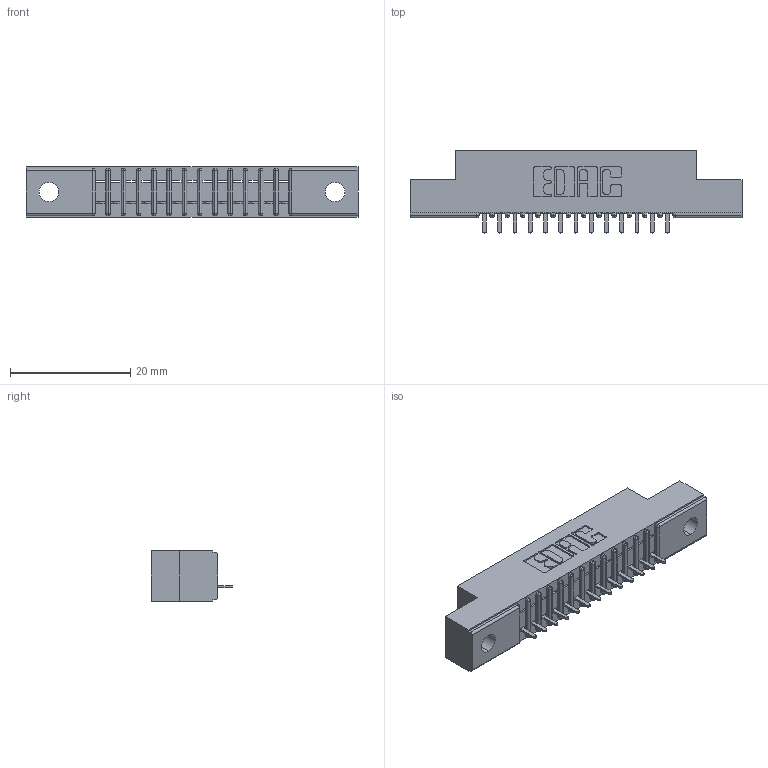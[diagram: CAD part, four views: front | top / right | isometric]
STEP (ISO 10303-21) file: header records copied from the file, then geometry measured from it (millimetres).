
FILE_DESCRIPTION (( 'STEP AP203' ), '1' );
FILE_NAME ('391-013-524-102.STEP', '2018-08-08T16:52:36', ( '' ), ( '' ), 'SwSTEP 2.0', 'SolidWorks 2016', '' );
FILE_SCHEMA (( 'CONFIG_CONTROL_DESIGN' ));
Length unit declared in the file: inch
Products named in the file (3): 391-013-524-102; 341 Part_.128 (3.25) Dia Mounting Holes; 341-292-001_341-292-124
Assembly tree (14 placements, depth 2):
  391-013-524-102
    341 Part_.128 (3.25) Dia Mounting Holes
    341-292-001_341-292-124  x13
Bounding box: 55.24 x 13.64 x 8.38 mm (x, y, z)
Volume: 3035.3 mm3; surface area: 4885.9 mm2
Topology: 14 solids, 14 shells, 1182 faces, 3397 edges, 2182 vertices
Faces by surface type: plane 731, cylinder 399, sphere 28, torus 24
Entity records: 19182 total; most frequent: CARTESIAN_POINT 3246, ORIENTED_EDGE 3234, DIRECTION 3157, EDGE_CURVE 1617, LINE 1275, VECTOR 1275, VERTEX_POINT 1030, AXIS2_PLACEMENT_3D 941
